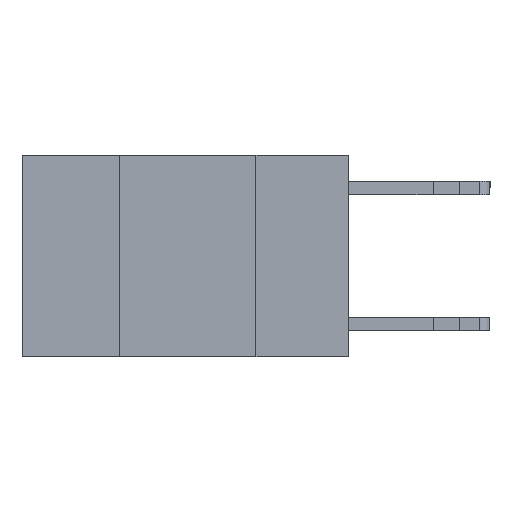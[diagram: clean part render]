
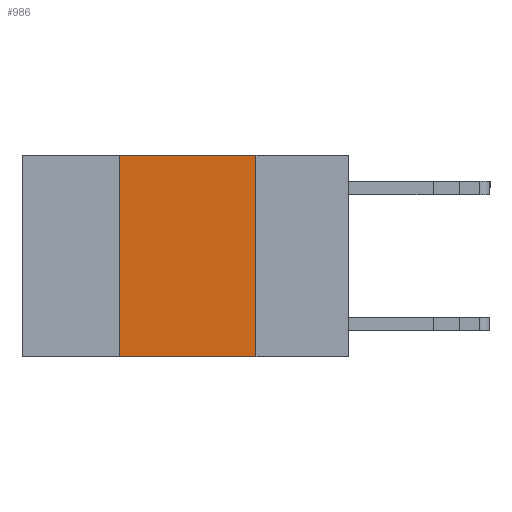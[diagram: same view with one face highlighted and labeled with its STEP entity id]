
A CAD part, left-side view. The second image highlights one B-rep face of the part: STEP entity #986.
In plain terms, the highlighted planar face has unit normal (-1, 0, 0).
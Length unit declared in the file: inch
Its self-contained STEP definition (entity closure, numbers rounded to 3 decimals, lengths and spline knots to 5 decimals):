
#986 = ADVANCED_FACE ( 'NONE', ( #12048 ), #15238, .F. ) ;
#1138 = DIRECTION ( 'NONE',  ( 0., -1., 0. ) ) ;
#1262 = VERTEX_POINT ( 'NONE', #3480 ) ;
#1916 = EDGE_CURVE ( 'NONE', #1262, #2199, #17876, .T. ) ;
#2028 = VECTOR ( 'NONE', #1138, 39.37008 ) ;
#2199 = VERTEX_POINT ( 'NONE', #12876 ) ;
#2371 = EDGE_CURVE ( 'NONE', #8904, #2199, #8978, .T. ) ;
#3480 = CARTESIAN_POINT ( 'NONE',  ( 0., 0.17, 0. ) ) ;
#4312 = CARTESIAN_POINT ( 'NONE',  ( 0., 0.6, 0. ) ) ;
#4368 = DIRECTION ( 'NONE',  ( 1., 0., 0. ) ) ;
#4961 = AXIS2_PLACEMENT_3D ( 'NONE', #6164, #4368, #5962 ) ;
#5490 = DIRECTION ( 'NONE',  ( 0., 0., 1. ) ) ;
#5781 = CARTESIAN_POINT ( 'NONE',  ( 0., 0.42, 0. ) ) ;
#5962 = DIRECTION ( 'NONE',  ( 0., 0., -1. ) ) ;
#6097 = ORIENTED_EDGE ( 'NONE', *, *, #9805, .F. ) ;
#6164 = CARTESIAN_POINT ( 'NONE',  ( 0., 0.6, 0. ) ) ;
#6289 = VECTOR ( 'NONE', #6974, 39.37008 ) ;
#6780 = EDGE_LOOP ( 'NONE', ( #9172, #17739, #6097, #13348 ) ) ;
#6974 = DIRECTION ( 'NONE',  ( 0., -1., 0. ) ) ;
#7724 = EDGE_CURVE ( 'NONE', #14312, #1262, #8919, .T. ) ;
#8800 = CARTESIAN_POINT ( 'NONE',  ( 0., 0.17, 0. ) ) ;
#8904 = VERTEX_POINT ( 'NONE', #14651 ) ;
#8919 = LINE ( 'NONE', #4312, #2028 ) ;
#8978 = LINE ( 'NONE', #15050, #6289 ) ;
#8999 = DIRECTION ( 'NONE',  ( 0., 0., -1. ) ) ;
#9172 = ORIENTED_EDGE ( 'NONE', *, *, #1916, .F. ) ;
#9805 = EDGE_CURVE ( 'NONE', #8904, #14312, #16463, .T. ) ;
#12048 = FACE_OUTER_BOUND ( 'NONE', #6780, .T. ) ;
#12876 = CARTESIAN_POINT ( 'NONE',  ( 0., 0.17, -0.37 ) ) ;
#13348 = ORIENTED_EDGE ( 'NONE', *, *, #2371, .T. ) ;
#14312 = VERTEX_POINT ( 'NONE', #19092 ) ;
#14651 = CARTESIAN_POINT ( 'NONE',  ( 0., 0.42, -0.37 ) ) ;
#15050 = CARTESIAN_POINT ( 'NONE',  ( 0., 0.6, -0.37 ) ) ;
#15238 = PLANE ( 'NONE',  #4961 ) ;
#16463 = LINE ( 'NONE', #5781, #18846 ) ;
#17739 = ORIENTED_EDGE ( 'NONE', *, *, #7724, .F. ) ;
#17876 = LINE ( 'NONE', #8800, #18392 ) ;
#18392 = VECTOR ( 'NONE', #8999, 39.37008 ) ;
#18846 = VECTOR ( 'NONE', #5490, 39.37008 ) ;
#19092 = CARTESIAN_POINT ( 'NONE',  ( 0., 0.42, 0. ) ) ;
